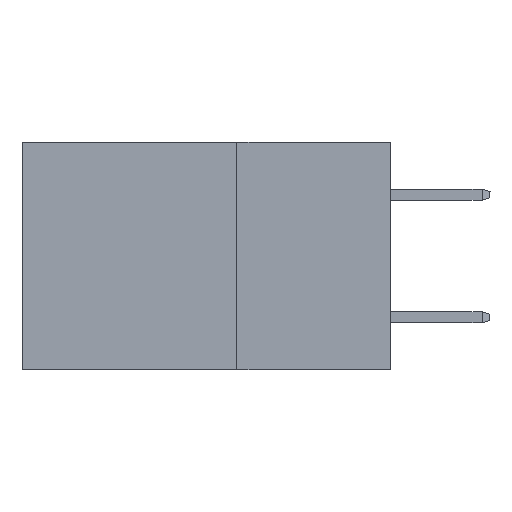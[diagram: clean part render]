
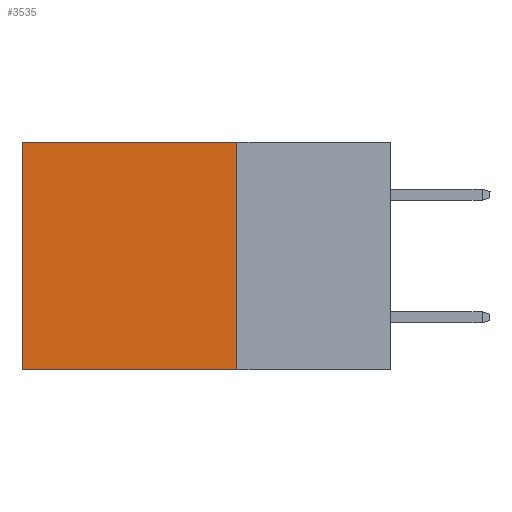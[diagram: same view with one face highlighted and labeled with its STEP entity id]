
A CAD part, left-side view. The second image highlights one B-rep face of the part: STEP entity #3535.
In plain terms, the highlighted planar face has unit normal (-1, 0, 0).
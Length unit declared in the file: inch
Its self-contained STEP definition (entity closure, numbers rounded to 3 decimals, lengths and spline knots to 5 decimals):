
#337 = FACE_OUTER_BOUND ( 'NONE', #7960, .T. ) ;
#517 = AXIS2_PLACEMENT_3D ( 'NONE', #7989, #6166, #5988 ) ;
#677 = VECTOR ( 'NONE', #9861, 39.37008 ) ;
#867 = EDGE_CURVE ( 'NONE', #962, #4847, #4332, .T. ) ;
#962 = VERTEX_POINT ( 'NONE', #9067 ) ;
#1210 = EDGE_CURVE ( 'NONE', #962, #1996, #10873, .T. ) ;
#1996 = VERTEX_POINT ( 'NONE', #9699 ) ;
#2408 = LINE ( 'NONE', #8023, #4812 ) ;
#2485 = ORIENTED_EDGE ( 'NONE', *, *, #8058, .T. ) ;
#3014 = VECTOR ( 'NONE', #6299, 39.37008 ) ;
#3323 = LINE ( 'NONE', #5257, #3014 ) ;
#3325 = ORIENTED_EDGE ( 'NONE', *, *, #9125, .F. ) ;
#3535 = ADVANCED_FACE ( 'NONE', ( #337 ), #7010, .F. ) ;
#4332 = LINE ( 'NONE', #5804, #11291 ) ;
#4423 = CARTESIAN_POINT ( 'NONE',  ( 0.2875, 0.6, -0.37 ) ) ;
#4757 = CARTESIAN_POINT ( 'NONE',  ( 0.2875, 0.6, 0. ) ) ;
#4812 = VECTOR ( 'NONE', #6183, 39.37008 ) ;
#4847 = VERTEX_POINT ( 'NONE', #4757 ) ;
#4866 = VERTEX_POINT ( 'NONE', #4423 ) ;
#5257 = CARTESIAN_POINT ( 'NONE',  ( 0.2875, 0.25, -0.37 ) ) ;
#5804 = CARTESIAN_POINT ( 'NONE',  ( 0.2875, 0.25, 0. ) ) ;
#5988 = DIRECTION ( 'NONE',  ( 0., 0., -1. ) ) ;
#6166 = DIRECTION ( 'NONE',  ( 1., 0., 0. ) ) ;
#6183 = DIRECTION ( 'NONE',  ( 0., 0., -1. ) ) ;
#6299 = DIRECTION ( 'NONE',  ( 0., 1., 0. ) ) ;
#6839 = CARTESIAN_POINT ( 'NONE',  ( 0.2875, 0.25, 0. ) ) ;
#7010 = PLANE ( 'NONE',  #517 ) ;
#7757 = ORIENTED_EDGE ( 'NONE', *, *, #1210, .F. ) ;
#7960 = EDGE_LOOP ( 'NONE', ( #2485, #3325, #7757, #9223 ) ) ;
#7989 = CARTESIAN_POINT ( 'NONE',  ( 0.2875, 0.25, 0. ) ) ;
#8023 = CARTESIAN_POINT ( 'NONE',  ( 0.2875, 0.6, 0. ) ) ;
#8058 = EDGE_CURVE ( 'NONE', #4847, #4866, #2408, .T. ) ;
#9067 = CARTESIAN_POINT ( 'NONE',  ( 0.2875, 0.25, 0. ) ) ;
#9125 = EDGE_CURVE ( 'NONE', #1996, #4866, #3323, .T. ) ;
#9223 = ORIENTED_EDGE ( 'NONE', *, *, #867, .T. ) ;
#9699 = CARTESIAN_POINT ( 'NONE',  ( 0.2875, 0.25, -0.37 ) ) ;
#9861 = DIRECTION ( 'NONE',  ( 0., 0., -1. ) ) ;
#10719 = DIRECTION ( 'NONE',  ( 0., 1., 0. ) ) ;
#10873 = LINE ( 'NONE', #6839, #677 ) ;
#11291 = VECTOR ( 'NONE', #10719, 39.37008 ) ;
